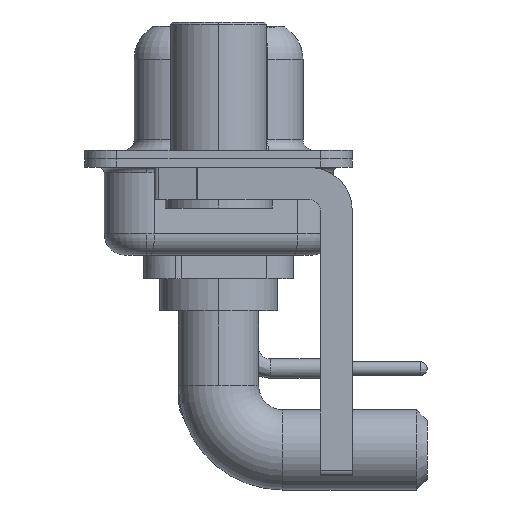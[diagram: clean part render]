
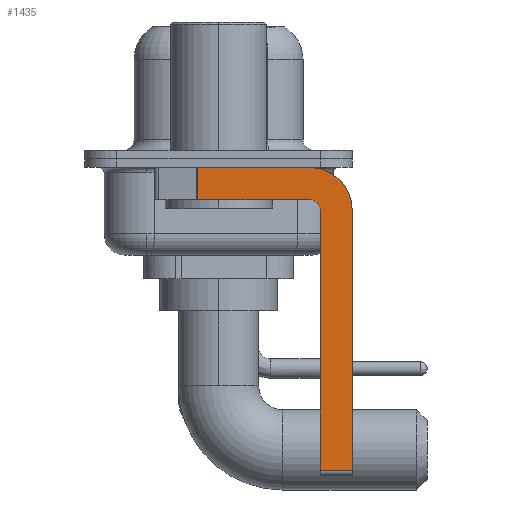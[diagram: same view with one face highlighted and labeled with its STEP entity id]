
A CAD part, left-side view. The second image highlights one B-rep face of the part: STEP entity #1435.
In plain terms, the highlighted planar face has unit normal (-1, 0, 0).
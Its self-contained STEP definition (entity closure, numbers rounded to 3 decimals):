
#122 = CARTESIAN_POINT ( 'NONE',  ( -2.9, 3., -0.4 ) ) ;
#168 = CARTESIAN_POINT ( 'NONE',  ( -2.9, 0.978, -0.4 ) ) ;
#343 = DIRECTION ( 'NONE',  ( 0., 0., -1. ) ) ;
#951 = DIRECTION ( 'NONE',  ( 1., 0., 0. ) ) ;
#1380 = LINE ( 'NONE', #122, #6630 ) ;
#1435 = ADVANCED_FACE ( 'NONE', ( #2364 ), #19253, .F. ) ;
#1526 = CARTESIAN_POINT ( 'NONE',  ( -2.9, -4.25, -1.9 ) ) ;
#1745 = CARTESIAN_POINT ( 'NONE',  ( -2.9, -6.25, -2.4 ) ) ;
#2019 = DIRECTION ( 'NONE',  ( 0., -1., 0. ) ) ;
#2262 = AXIS2_PLACEMENT_3D ( 'NONE', #5443, #951, #9863 ) ;
#2282 = ORIENTED_EDGE ( 'NONE', *, *, #14567, .F. ) ;
#2302 = CARTESIAN_POINT ( 'NONE',  ( -2.9, 0.978, -1.9 ) ) ;
#2364 = FACE_OUTER_BOUND ( 'NONE', #11765, .T. ) ;
#2637 = VERTEX_POINT ( 'NONE', #3654 ) ;
#2713 = CARTESIAN_POINT ( 'NONE',  ( -2.9, -4.25, -0.4 ) ) ;
#3213 = AXIS2_PLACEMENT_3D ( 'NONE', #10722, #16740, #13597 ) ;
#3654 = CARTESIAN_POINT ( 'NONE',  ( -2.9, -6.25, -2.4 ) ) ;
#4127 = VERTEX_POINT ( 'NONE', #168 ) ;
#4224 = CARTESIAN_POINT ( 'NONE',  ( -2.9, -4.25, -2.4 ) ) ;
#4620 = DIRECTION ( 'NONE',  ( 0., -1., 0. ) ) ;
#4656 = LINE ( 'NONE', #7787, #14286 ) ;
#5120 = EDGE_CURVE ( 'NONE', #4127, #18490, #4656, .T. ) ;
#5293 = ORIENTED_EDGE ( 'NONE', *, *, #16993, .F. ) ;
#5443 = CARTESIAN_POINT ( 'NONE',  ( -2.9, -4.25, -2.4 ) ) ;
#5737 = ORIENTED_EDGE ( 'NONE', *, *, #10637, .T. ) ;
#6227 = CARTESIAN_POINT ( 'NONE',  ( -2.9, -4.75, -14.8 ) ) ;
#6304 = VERTEX_POINT ( 'NONE', #1526 ) ;
#6368 = VERTEX_POINT ( 'NONE', #2713 ) ;
#6508 = ORIENTED_EDGE ( 'NONE', *, *, #13395, .F. ) ;
#6630 = VECTOR ( 'NONE', #4620, 1000. ) ;
#7186 = VECTOR ( 'NONE', #2019, 1000. ) ;
#7267 = VERTEX_POINT ( 'NONE', #18592 ) ;
#7334 = VERTEX_POINT ( 'NONE', #8354 ) ;
#7607 = LINE ( 'NONE', #6227, #8539 ) ;
#7787 = CARTESIAN_POINT ( 'NONE',  ( -2.9, 0.978, -1.9 ) ) ;
#7943 = AXIS2_PLACEMENT_3D ( 'NONE', #4224, #15997, #17284 ) ;
#8354 = CARTESIAN_POINT ( 'NONE',  ( -2.9, -4.75, -2.4 ) ) ;
#8539 = VECTOR ( 'NONE', #10623, 1000. ) ;
#9192 = DIRECTION ( 'NONE',  ( 0., 0., -1. ) ) ;
#9458 = CIRCLE ( 'NONE', #2262, 2. ) ;
#9471 = VECTOR ( 'NONE', #9192, 1000. ) ;
#9863 = DIRECTION ( 'NONE',  ( 0., 0., -1. ) ) ;
#10578 = ORIENTED_EDGE ( 'NONE', *, *, #10801, .F. ) ;
#10623 = DIRECTION ( 'NONE',  ( 0., 0., 1. ) ) ;
#10637 = EDGE_CURVE ( 'NONE', #15456, #7267, #12319, .T. ) ;
#10702 = CARTESIAN_POINT ( 'NONE',  ( -2.9, -4.75, -14.55 ) ) ;
#10722 = CARTESIAN_POINT ( 'NONE',  ( -2.9, -4.25, -2.4 ) ) ;
#10801 = EDGE_CURVE ( 'NONE', #6304, #18490, #18916, .T. ) ;
#11154 = ORIENTED_EDGE ( 'NONE', *, *, #5120, .T. ) ;
#11411 = CARTESIAN_POINT ( 'NONE',  ( -2.9, -4.25, -1.9 ) ) ;
#11765 = EDGE_LOOP ( 'NONE', ( #2282, #11154, #10578, #19070, #5293, #5737, #18354, #6508 ) ) ;
#12319 = LINE ( 'NONE', #18332, #7186 ) ;
#13395 = EDGE_CURVE ( 'NONE', #6368, #2637, #9458, .T. ) ;
#13512 = LINE ( 'NONE', #1745, #9471 ) ;
#13597 = DIRECTION ( 'NONE',  ( 0., 0., 1. ) ) ;
#13659 = EDGE_CURVE ( 'NONE', #7334, #6304, #16687, .T. ) ;
#14286 = VECTOR ( 'NONE', #343, 1000. ) ;
#14567 = EDGE_CURVE ( 'NONE', #4127, #6368, #1380, .T. ) ;
#15456 = VERTEX_POINT ( 'NONE', #10702 ) ;
#15997 = DIRECTION ( 'NONE',  ( 1., 0., 0. ) ) ;
#16526 = EDGE_CURVE ( 'NONE', #2637, #7267, #13512, .T. ) ;
#16687 = CIRCLE ( 'NONE', #3213, 0.5 ) ;
#16740 = DIRECTION ( 'NONE',  ( -1., 0., 0. ) ) ;
#16993 = EDGE_CURVE ( 'NONE', #15456, #7334, #7607, .T. ) ;
#17284 = DIRECTION ( 'NONE',  ( 0., 0., -1. ) ) ;
#17432 = DIRECTION ( 'NONE',  ( 0., 1., 0. ) ) ;
#18332 = CARTESIAN_POINT ( 'NONE',  ( -2.9, -4.25, -14.55 ) ) ;
#18354 = ORIENTED_EDGE ( 'NONE', *, *, #16526, .F. ) ;
#18490 = VERTEX_POINT ( 'NONE', #2302 ) ;
#18514 = VECTOR ( 'NONE', #17432, 1000. ) ;
#18592 = CARTESIAN_POINT ( 'NONE',  ( -2.9, -6.25, -14.55 ) ) ;
#18916 = LINE ( 'NONE', #11411, #18514 ) ;
#19070 = ORIENTED_EDGE ( 'NONE', *, *, #13659, .F. ) ;
#19253 = PLANE ( 'NONE',  #7943 ) ;
